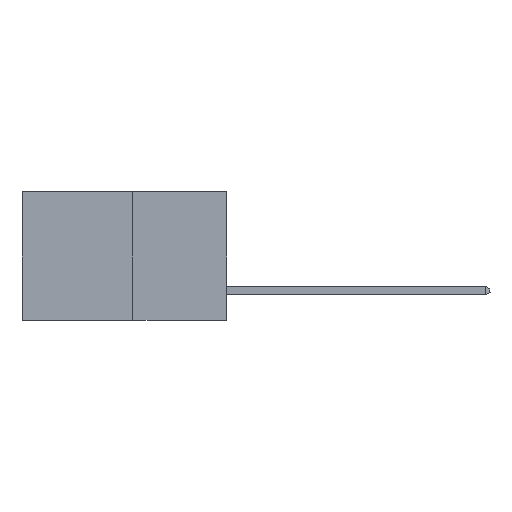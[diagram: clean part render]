
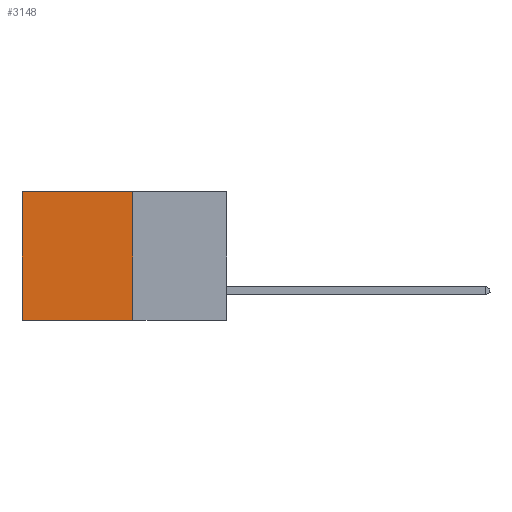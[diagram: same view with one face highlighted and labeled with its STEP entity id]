
A CAD part, left-side view. The second image highlights one B-rep face of the part: STEP entity #3148.
In plain terms, the highlighted planar face has unit normal (-1, 0, 0).
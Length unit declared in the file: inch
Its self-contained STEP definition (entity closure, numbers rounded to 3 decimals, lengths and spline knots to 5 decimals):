
#159 = EDGE_LOOP ( 'NONE', ( #7197, #12937, #2881, #3559 ) ) ;
#277 = CARTESIAN_POINT ( 'NONE',  ( 0.277, 0.59, -0.37 ) ) ;
#319 = VECTOR ( 'NONE', #2664, 39.37008 ) ;
#444 = VERTEX_POINT ( 'NONE', #9310 ) ;
#665 = LINE ( 'NONE', #1548, #319 ) ;
#812 = CARTESIAN_POINT ( 'NONE',  ( 0.277, 0.27, -0.37 ) ) ;
#1548 = CARTESIAN_POINT ( 'NONE',  ( 0.277, 0.27, -0.37 ) ) ;
#1832 = LINE ( 'NONE', #8231, #4058 ) ;
#1935 = DIRECTION ( 'NONE',  ( 0., 0., -1. ) ) ;
#2404 = VECTOR ( 'NONE', #7787, 39.37008 ) ;
#2664 = DIRECTION ( 'NONE',  ( 0., 1., 0. ) ) ;
#2877 = LINE ( 'NONE', #9997, #5397 ) ;
#2881 = ORIENTED_EDGE ( 'NONE', *, *, #11329, .F. ) ;
#2934 = DIRECTION ( 'NONE',  ( 0., 0., -1. ) ) ;
#3103 = AXIS2_PLACEMENT_3D ( 'NONE', #812, #8291, #1935 ) ;
#3148 = ADVANCED_FACE ( 'NONE', ( #5796 ), #9306, .F. ) ;
#3196 = CARTESIAN_POINT ( 'NONE',  ( 0.277, 0.27, -0.37 ) ) ;
#3353 = EDGE_CURVE ( 'NONE', #10932, #4485, #13473, .T. ) ;
#3559 = ORIENTED_EDGE ( 'NONE', *, *, #11657, .T. ) ;
#3761 = VERTEX_POINT ( 'NONE', #3196 ) ;
#4058 = VECTOR ( 'NONE', #2934, 39.37008 ) ;
#4297 = CARTESIAN_POINT ( 'NONE',  ( 0.277, 0.59, -0.37 ) ) ;
#4485 = VERTEX_POINT ( 'NONE', #4297 ) ;
#4603 = EDGE_CURVE ( 'NONE', #3761, #4485, #665, .T. ) ;
#5397 = VECTOR ( 'NONE', #6863, 39.37008 ) ;
#5796 = FACE_OUTER_BOUND ( 'NONE', #159, .T. ) ;
#6863 = DIRECTION ( 'NONE',  ( 0., 1., 0. ) ) ;
#7197 = ORIENTED_EDGE ( 'NONE', *, *, #3353, .T. ) ;
#7787 = DIRECTION ( 'NONE',  ( 0., 0., -1. ) ) ;
#8231 = CARTESIAN_POINT ( 'NONE',  ( 0.277, 0.27, -0.37 ) ) ;
#8291 = DIRECTION ( 'NONE',  ( 1., 0., 0. ) ) ;
#8629 = CARTESIAN_POINT ( 'NONE',  ( 0.277, 0.59, 0. ) ) ;
#9306 = PLANE ( 'NONE',  #3103 ) ;
#9310 = CARTESIAN_POINT ( 'NONE',  ( 0.277, 0.27, 0. ) ) ;
#9997 = CARTESIAN_POINT ( 'NONE',  ( 0.277, 0.27, 0. ) ) ;
#10932 = VERTEX_POINT ( 'NONE', #8629 ) ;
#11329 = EDGE_CURVE ( 'NONE', #444, #3761, #1832, .T. ) ;
#11657 = EDGE_CURVE ( 'NONE', #444, #10932, #2877, .T. ) ;
#12937 = ORIENTED_EDGE ( 'NONE', *, *, #4603, .F. ) ;
#13473 = LINE ( 'NONE', #277, #2404 ) ;
